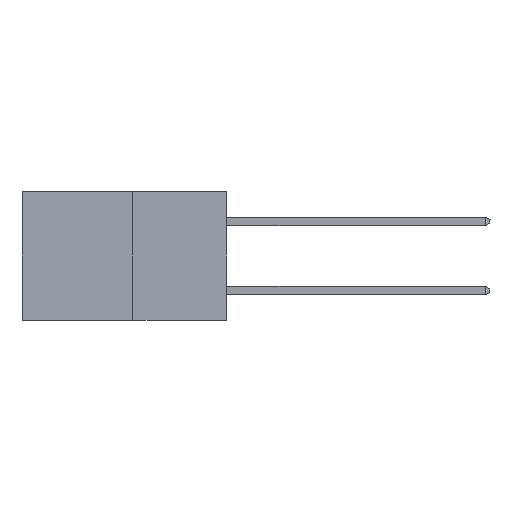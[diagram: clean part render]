
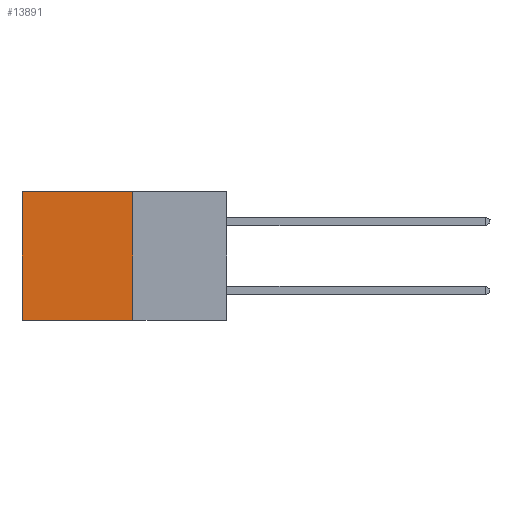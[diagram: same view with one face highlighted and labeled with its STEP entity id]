
A CAD part, left-side view. The second image highlights one B-rep face of the part: STEP entity #13891.
In plain terms, the highlighted planar face has unit normal (-1, 0, 0).
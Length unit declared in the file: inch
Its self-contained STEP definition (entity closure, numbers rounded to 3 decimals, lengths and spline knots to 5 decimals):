
#105 = LINE ( 'NONE', #6263, #14214 ) ;
#985 = VERTEX_POINT ( 'NONE', #9757 ) ;
#1526 = PLANE ( 'NONE',  #9508 ) ;
#1577 = DIRECTION ( 'NONE',  ( 0., 0., -1. ) ) ;
#2086 = EDGE_CURVE ( 'NONE', #12956, #10346, #105, .T. ) ;
#2202 = ORIENTED_EDGE ( 'NONE', *, *, #10909, .T. ) ;
#3040 = CARTESIAN_POINT ( 'NONE',  ( 0.277, 0.27, 0. ) ) ;
#4170 = CARTESIAN_POINT ( 'NONE',  ( 0.277, 0.27, 0. ) ) ;
#5307 = VECTOR ( 'NONE', #8654, 39.37008 ) ;
#5355 = DIRECTION ( 'NONE',  ( 0., 0., -1. ) ) ;
#5819 = EDGE_CURVE ( 'NONE', #12327, #12956, #13309, .T. ) ;
#6229 = LINE ( 'NONE', #13050, #13163 ) ;
#6263 = CARTESIAN_POINT ( 'NONE',  ( 0.277, 0.27, -0.37 ) ) ;
#7117 = CARTESIAN_POINT ( 'NONE',  ( 0.277, 0.27, -0.37 ) ) ;
#7564 = DIRECTION ( 'NONE',  ( 0., 1., 0. ) ) ;
#8247 = DIRECTION ( 'NONE',  ( 1., 0., 0. ) ) ;
#8654 = DIRECTION ( 'NONE',  ( 0., 1., 0. ) ) ;
#8830 = EDGE_CURVE ( 'NONE', #985, #10346, #6229, .T. ) ;
#8919 = CARTESIAN_POINT ( 'NONE',  ( 0.277, 0.59, -0.37 ) ) ;
#9020 = CARTESIAN_POINT ( 'NONE',  ( 0.277, 0.27, -0.37 ) ) ;
#9169 = DIRECTION ( 'NONE',  ( 0., 0., -1. ) ) ;
#9508 = AXIS2_PLACEMENT_3D ( 'NONE', #7117, #8247, #1577 ) ;
#9704 = VECTOR ( 'NONE', #9169, 39.37008 ) ;
#9757 = CARTESIAN_POINT ( 'NONE',  ( 0.277, 0.59, 0. ) ) ;
#10047 = ORIENTED_EDGE ( 'NONE', *, *, #2086, .F. ) ;
#10346 = VERTEX_POINT ( 'NONE', #8919 ) ;
#10909 = EDGE_CURVE ( 'NONE', #12327, #985, #14099, .T. ) ;
#11001 = FACE_OUTER_BOUND ( 'NONE', #11867, .T. ) ;
#11867 = EDGE_LOOP ( 'NONE', ( #11948, #10047, #13304, #2202 ) ) ;
#11948 = ORIENTED_EDGE ( 'NONE', *, *, #8830, .T. ) ;
#12135 = CARTESIAN_POINT ( 'NONE',  ( 0.277, 0.27, -0.37 ) ) ;
#12327 = VERTEX_POINT ( 'NONE', #3040 ) ;
#12956 = VERTEX_POINT ( 'NONE', #12135 ) ;
#13050 = CARTESIAN_POINT ( 'NONE',  ( 0.277, 0.59, -0.37 ) ) ;
#13163 = VECTOR ( 'NONE', #5355, 39.37008 ) ;
#13304 = ORIENTED_EDGE ( 'NONE', *, *, #5819, .F. ) ;
#13309 = LINE ( 'NONE', #9020, #9704 ) ;
#13891 = ADVANCED_FACE ( 'NONE', ( #11001 ), #1526, .F. ) ;
#14099 = LINE ( 'NONE', #4170, #5307 ) ;
#14214 = VECTOR ( 'NONE', #7564, 39.37008 ) ;
